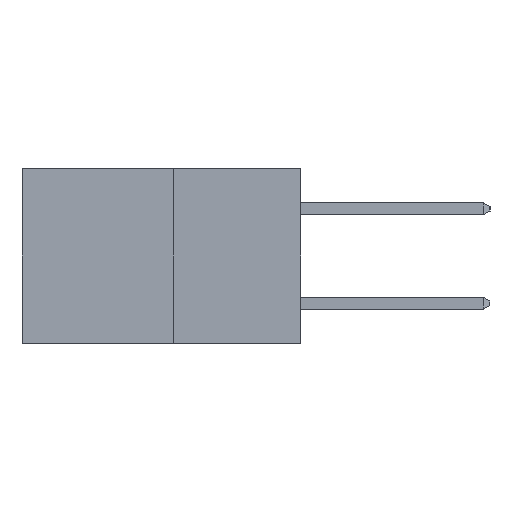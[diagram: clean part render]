
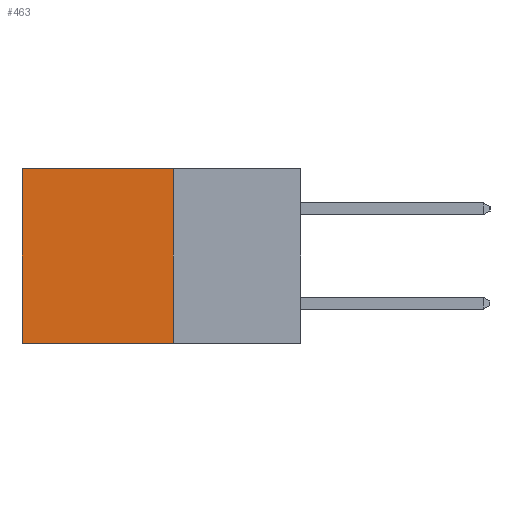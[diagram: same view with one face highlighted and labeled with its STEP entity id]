
A CAD part, left-side view. The second image highlights one B-rep face of the part: STEP entity #463.
In plain terms, the highlighted planar face has unit normal (-1, 0, 0).
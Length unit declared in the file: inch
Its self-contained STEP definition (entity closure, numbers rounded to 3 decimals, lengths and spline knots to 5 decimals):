
#463 = ADVANCED_FACE ( 'NONE', ( #9018 ), #7551, .F. ) ;
#469 = LINE ( 'NONE', #4205, #5081 ) ;
#659 = EDGE_CURVE ( 'NONE', #6890, #1534, #6503, .T. ) ;
#707 = EDGE_CURVE ( 'NONE', #6003, #7283, #6232, .T. ) ;
#1416 = CARTESIAN_POINT ( 'NONE',  ( 0.277, 0.59, -0.37 ) ) ;
#1534 = VERTEX_POINT ( 'NONE', #9045 ) ;
#1601 = ORIENTED_EDGE ( 'NONE', *, *, #659, .F. ) ;
#1798 = VECTOR ( 'NONE', #2333, 39.37008 ) ;
#1976 = EDGE_CURVE ( 'NONE', #1534, #7283, #6204, .T. ) ;
#2214 = CARTESIAN_POINT ( 'NONE',  ( 0.277, 0.27, -0.37 ) ) ;
#2333 = DIRECTION ( 'NONE',  ( 0., 0., -1. ) ) ;
#2786 = AXIS2_PLACEMENT_3D ( 'NONE', #8875, #8873, #7986 ) ;
#3755 = ORIENTED_EDGE ( 'NONE', *, *, #707, .T. ) ;
#3898 = VECTOR ( 'NONE', #4088, 39.37008 ) ;
#4028 = ORIENTED_EDGE ( 'NONE', *, *, #10800, .T. ) ;
#4088 = DIRECTION ( 'NONE',  ( 0., 1., 0. ) ) ;
#4205 = CARTESIAN_POINT ( 'NONE',  ( 0.277, 0.27, 0. ) ) ;
#4465 = CARTESIAN_POINT ( 'NONE',  ( 0.277, 0.27, -0.37 ) ) ;
#5081 = VECTOR ( 'NONE', #11243, 39.37008 ) ;
#5118 = EDGE_LOOP ( 'NONE', ( #3755, #6054, #1601, #4028 ) ) ;
#6003 = VERTEX_POINT ( 'NONE', #9909 ) ;
#6054 = ORIENTED_EDGE ( 'NONE', *, *, #1976, .F. ) ;
#6107 = CARTESIAN_POINT ( 'NONE',  ( 0.277, 0.27, 0. ) ) ;
#6204 = LINE ( 'NONE', #4465, #3898 ) ;
#6232 = LINE ( 'NONE', #8425, #10396 ) ;
#6503 = LINE ( 'NONE', #2214, #1798 ) ;
#6890 = VERTEX_POINT ( 'NONE', #6107 ) ;
#7283 = VERTEX_POINT ( 'NONE', #1416 ) ;
#7551 = PLANE ( 'NONE',  #2786 ) ;
#7986 = DIRECTION ( 'NONE',  ( 0., 0., -1. ) ) ;
#8425 = CARTESIAN_POINT ( 'NONE',  ( 0.277, 0.59, -0.37 ) ) ;
#8631 = DIRECTION ( 'NONE',  ( 0., 0., -1. ) ) ;
#8873 = DIRECTION ( 'NONE',  ( 1., 0., 0. ) ) ;
#8875 = CARTESIAN_POINT ( 'NONE',  ( 0.277, 0.27, -0.37 ) ) ;
#9018 = FACE_OUTER_BOUND ( 'NONE', #5118, .T. ) ;
#9045 = CARTESIAN_POINT ( 'NONE',  ( 0.277, 0.27, -0.37 ) ) ;
#9909 = CARTESIAN_POINT ( 'NONE',  ( 0.277, 0.59, 0. ) ) ;
#10396 = VECTOR ( 'NONE', #8631, 39.37008 ) ;
#10800 = EDGE_CURVE ( 'NONE', #6890, #6003, #469, .T. ) ;
#11243 = DIRECTION ( 'NONE',  ( 0., 1., 0. ) ) ;
